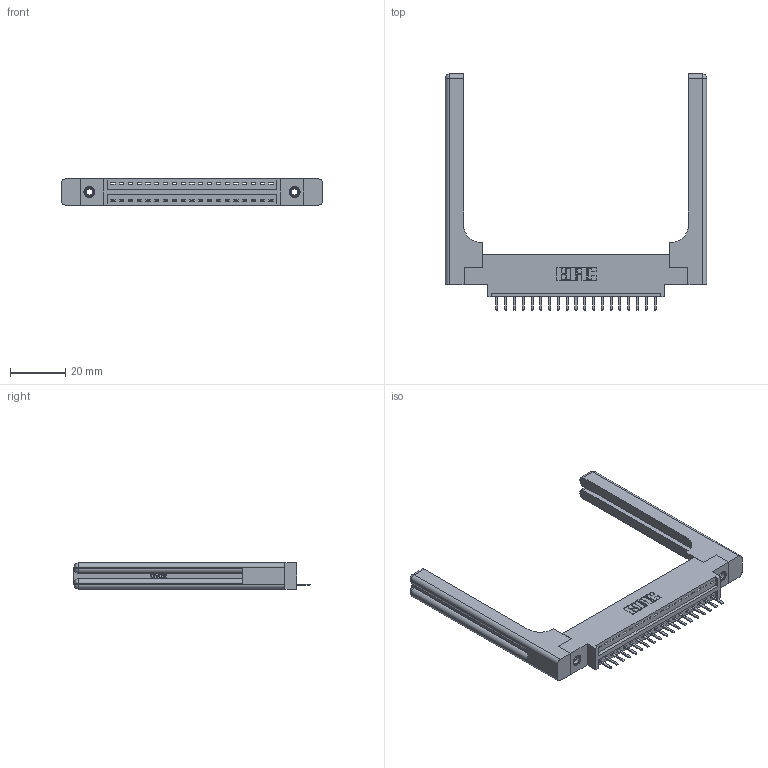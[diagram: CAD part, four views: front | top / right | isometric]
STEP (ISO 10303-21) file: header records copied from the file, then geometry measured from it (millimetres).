
FILE_DESCRIPTION (( 'STEP AP203' ), '1' );
FILE_NAME ('346-019-520-658.STEP', '2022-05-05T15:02:20', ( '' ), ( '' ), 'SwSTEP 2.0', 'SolidWorks 2020', '' );
FILE_SCHEMA (( 'CONFIG_CONTROL_DESIGN' ));
Length unit declared in the file: inch
Products named in the file (5): 345-250-001_345-250-001-102; 346 Part_0.170 Offset - 0.156 Dia-TH; 346-019-520-658; 345-292-001_345-293-120; 346-220-058_345-220-058
Assembly tree (24 placements, depth 2):
  346-019-520-658
    346 Part_0.170 Offset - 0.156 Dia-TH
    345-292-001_345-293-120  x19
    345-250-001_345-250-001-102  x2
    346-220-058_345-220-058  x2
Bounding box: 94.39 x 85.29 x 9.4 mm (x, y, z)
Volume: 16167.4 mm3; surface area: 15741.7 mm2
Topology: 24 solids, 24 shells, 1574 faces, 4539 edges, 2954 vertices
Faces by surface type: plane 1040, cylinder 474, bspline 36, cone 12, sphere 8, torus 4
Entity records: 20732 total; most frequent: CARTESIAN_POINT 4556, ORIENTED_EDGE 3292, DIRECTION 2964, EDGE_CURVE 1646, LINE 1342, VECTOR 1342, VERTEX_POINT 1086, AXIS2_PLACEMENT_3D 811
